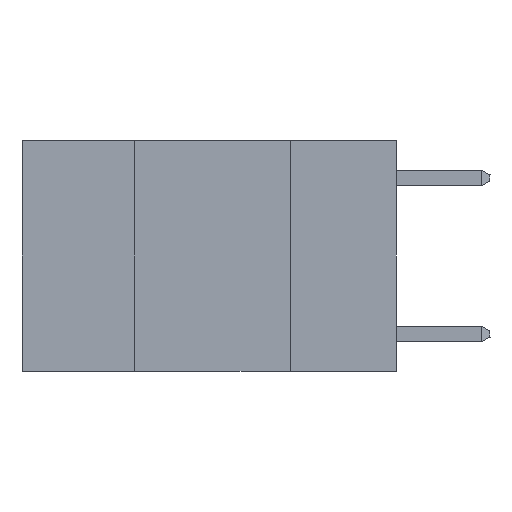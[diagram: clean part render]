
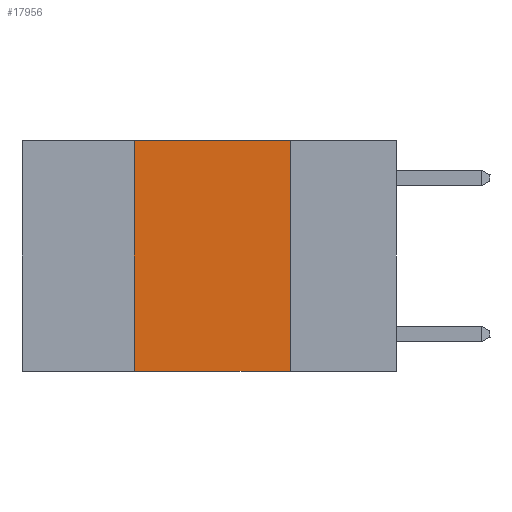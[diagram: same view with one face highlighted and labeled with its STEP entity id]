
A CAD part, left-side view. The second image highlights one B-rep face of the part: STEP entity #17956.
In plain terms, the highlighted planar face has unit normal (-1, 0, 0).
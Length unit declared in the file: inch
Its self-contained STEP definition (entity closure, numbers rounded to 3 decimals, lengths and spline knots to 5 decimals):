
#1165 = ORIENTED_EDGE ( 'NONE', *, *, #11569, .F. ) ;
#1740 = VECTOR ( 'NONE', #16718, 39.37008 ) ;
#2410 = VERTEX_POINT ( 'NONE', #6951 ) ;
#3275 = VERTEX_POINT ( 'NONE', #20989 ) ;
#3335 = CARTESIAN_POINT ( 'NONE',  ( 0., 0.6, 0. ) ) ;
#3629 = ORIENTED_EDGE ( 'NONE', *, *, #14352, .F. ) ;
#3678 = DIRECTION ( 'NONE',  ( 1., 0., 0. ) ) ;
#4227 = ORIENTED_EDGE ( 'NONE', *, *, #19449, .F. ) ;
#4318 = DIRECTION ( 'NONE',  ( 0., 0., -1. ) ) ;
#4794 = CARTESIAN_POINT ( 'NONE',  ( 0., 0.17, -0.37 ) ) ;
#5958 = AXIS2_PLACEMENT_3D ( 'NONE', #3335, #3678, #9060 ) ;
#5986 = CARTESIAN_POINT ( 'NONE',  ( 0., 0.17, 0. ) ) ;
#6457 = VERTEX_POINT ( 'NONE', #7906 ) ;
#6535 = LINE ( 'NONE', #9915, #1740 ) ;
#6951 = CARTESIAN_POINT ( 'NONE',  ( 0., 0.42, -0.37 ) ) ;
#7290 = DIRECTION ( 'NONE',  ( 0., 0., 1. ) ) ;
#7906 = CARTESIAN_POINT ( 'NONE',  ( 0., 0.42, 0. ) ) ;
#9060 = DIRECTION ( 'NONE',  ( 0., 0., -1. ) ) ;
#9082 = DIRECTION ( 'NONE',  ( 0., -1., 0. ) ) ;
#9290 = CARTESIAN_POINT ( 'NONE',  ( 0., 0.6, 0. ) ) ;
#9915 = CARTESIAN_POINT ( 'NONE',  ( 0., 0.6, -0.37 ) ) ;
#10357 = VECTOR ( 'NONE', #7290, 39.37008 ) ;
#10880 = VECTOR ( 'NONE', #4318, 39.37008 ) ;
#11064 = ORIENTED_EDGE ( 'NONE', *, *, #15113, .T. ) ;
#11569 = EDGE_CURVE ( 'NONE', #3275, #14598, #17501, .T. ) ;
#11961 = FACE_OUTER_BOUND ( 'NONE', #21727, .T. ) ;
#14352 = EDGE_CURVE ( 'NONE', #6457, #3275, #19559, .T. ) ;
#14598 = VERTEX_POINT ( 'NONE', #4794 ) ;
#15113 = EDGE_CURVE ( 'NONE', #2410, #14598, #6535, .T. ) ;
#16718 = DIRECTION ( 'NONE',  ( 0., -1., 0. ) ) ;
#17005 = VECTOR ( 'NONE', #9082, 39.37008 ) ;
#17453 = LINE ( 'NONE', #19038, #10357 ) ;
#17501 = LINE ( 'NONE', #5986, #10880 ) ;
#17956 = ADVANCED_FACE ( 'NONE', ( #11961 ), #20554, .F. ) ;
#19038 = CARTESIAN_POINT ( 'NONE',  ( 0., 0.42, 0. ) ) ;
#19449 = EDGE_CURVE ( 'NONE', #2410, #6457, #17453, .T. ) ;
#19559 = LINE ( 'NONE', #9290, #17005 ) ;
#20554 = PLANE ( 'NONE',  #5958 ) ;
#20989 = CARTESIAN_POINT ( 'NONE',  ( 0., 0.17, 0. ) ) ;
#21727 = EDGE_LOOP ( 'NONE', ( #1165, #3629, #4227, #11064 ) ) ;
